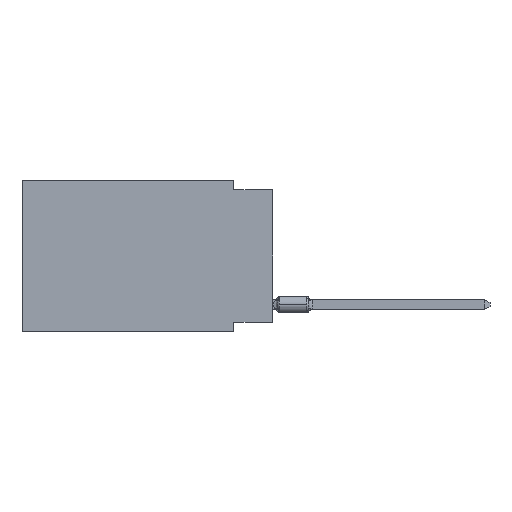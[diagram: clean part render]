
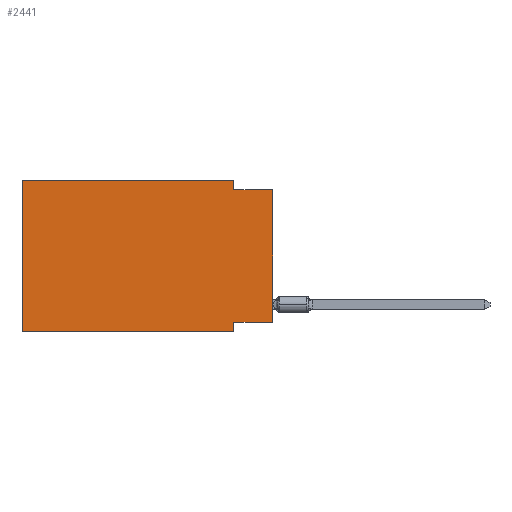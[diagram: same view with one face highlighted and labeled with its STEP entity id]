
A CAD part, left-side view. The second image highlights one B-rep face of the part: STEP entity #2441.
In plain terms, the highlighted planar face has unit normal (-1, 0, 0).
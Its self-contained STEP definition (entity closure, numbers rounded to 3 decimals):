
#49 = CARTESIAN_POINT ( 'NONE',  ( 0., 2.54, 0. ) ) ;
#598 = VECTOR ( 'NONE', #2566, 1000. ) ;
#626 = DIRECTION ( 'NONE',  ( 0., 1., 0. ) ) ;
#1036 = ORIENTED_EDGE ( 'NONE', *, *, #18846, .F. ) ;
#1478 = EDGE_LOOP ( 'NONE', ( #9304, #20825, #6450, #1036, #4518, #3928, #22401, #12254 ) ) ;
#2416 = CARTESIAN_POINT ( 'NONE',  ( 0., 16.383, 0. ) ) ;
#2441 = ADVANCED_FACE ( 'NONE', ( #10969 ), #17260, .F. ) ;
#2447 = CARTESIAN_POINT ( 'NONE',  ( 0., 16.383, -9.906 ) ) ;
#2566 = DIRECTION ( 'NONE',  ( 0., 0., 1. ) ) ;
#2582 = LINE ( 'NONE', #22959, #13742 ) ;
#3321 = DIRECTION ( 'NONE',  ( 0., -1., 0. ) ) ;
#3928 = ORIENTED_EDGE ( 'NONE', *, *, #16907, .T. ) ;
#4476 = VERTEX_POINT ( 'NONE', #7484 ) ;
#4518 = ORIENTED_EDGE ( 'NONE', *, *, #6548, .F. ) ;
#4574 = LINE ( 'NONE', #6696, #598 ) ;
#4639 = VECTOR ( 'NONE', #17729, 1000. ) ;
#4999 = VECTOR ( 'NONE', #14566, 1000. ) ;
#5098 = VERTEX_POINT ( 'NONE', #22165 ) ;
#5389 = LINE ( 'NONE', #21756, #4639 ) ;
#5683 = VECTOR ( 'NONE', #3321, 1000. ) ;
#6090 = EDGE_CURVE ( 'NONE', #9878, #5098, #6742, .T. ) ;
#6450 = ORIENTED_EDGE ( 'NONE', *, *, #26246, .F. ) ;
#6548 = EDGE_CURVE ( 'NONE', #11024, #13679, #7244, .T. ) ;
#6696 = CARTESIAN_POINT ( 'NONE',  ( 0., 0., 0. ) ) ;
#6742 = LINE ( 'NONE', #17210, #25086 ) ;
#6817 = DIRECTION ( 'NONE',  ( 0., -1., 0. ) ) ;
#7244 = LINE ( 'NONE', #23626, #4999 ) ;
#7484 = CARTESIAN_POINT ( 'NONE',  ( 0., 2.54, -0.635 ) ) ;
#7586 = LINE ( 'NONE', #21686, #5683 ) ;
#8890 = VERTEX_POINT ( 'NONE', #19800 ) ;
#9199 = DIRECTION ( 'NONE',  ( 0., 0., -1. ) ) ;
#9304 = ORIENTED_EDGE ( 'NONE', *, *, #19993, .T. ) ;
#9878 = VERTEX_POINT ( 'NONE', #22437 ) ;
#10745 = DIRECTION ( 'NONE',  ( 0., 0., -1. ) ) ;
#10830 = VERTEX_POINT ( 'NONE', #49 ) ;
#10969 = FACE_OUTER_BOUND ( 'NONE', #1478, .T. ) ;
#11024 = VERTEX_POINT ( 'NONE', #2447 ) ;
#12115 = EDGE_CURVE ( 'NONE', #4476, #24833, #5389, .T. ) ;
#12254 = ORIENTED_EDGE ( 'NONE', *, *, #6090, .F. ) ;
#13157 = LINE ( 'NONE', #15167, #19545 ) ;
#13679 = VERTEX_POINT ( 'NONE', #2416 ) ;
#13742 = VECTOR ( 'NONE', #10745, 1000. ) ;
#13767 = LINE ( 'NONE', #15892, #24077 ) ;
#14566 = DIRECTION ( 'NONE',  ( 0., 0., 1. ) ) ;
#15167 = CARTESIAN_POINT ( 'NONE',  ( 0., 16.383, 0. ) ) ;
#15392 = CARTESIAN_POINT ( 'NONE',  ( 0., 16.383, 0. ) ) ;
#15883 = AXIS2_PLACEMENT_3D ( 'NONE', #15392, #25186, #9199 ) ;
#15892 = CARTESIAN_POINT ( 'NONE',  ( 0., 2.54, -9.906 ) ) ;
#16907 = EDGE_CURVE ( 'NONE', #11024, #8890, #7586, .T. ) ;
#17210 = CARTESIAN_POINT ( 'NONE',  ( 0., 0., -9.271 ) ) ;
#17260 = PLANE ( 'NONE',  #15883 ) ;
#17729 = DIRECTION ( 'NONE',  ( 0., -1., 0. ) ) ;
#18846 = EDGE_CURVE ( 'NONE', #13679, #10830, #13157, .T. ) ;
#19545 = VECTOR ( 'NONE', #6817, 1000. ) ;
#19800 = CARTESIAN_POINT ( 'NONE',  ( 0., 2.54, -9.906 ) ) ;
#19904 = DIRECTION ( 'NONE',  ( 0., 0., -1. ) ) ;
#19993 = EDGE_CURVE ( 'NONE', #9878, #24833, #4574, .T. ) ;
#20825 = ORIENTED_EDGE ( 'NONE', *, *, #12115, .F. ) ;
#21686 = CARTESIAN_POINT ( 'NONE',  ( 0., 16.383, -9.906 ) ) ;
#21756 = CARTESIAN_POINT ( 'NONE',  ( 0., 0., -0.635 ) ) ;
#22165 = CARTESIAN_POINT ( 'NONE',  ( 0., 2.54, -9.271 ) ) ;
#22401 = ORIENTED_EDGE ( 'NONE', *, *, #24304, .F. ) ;
#22437 = CARTESIAN_POINT ( 'NONE',  ( 0., 0., -9.271 ) ) ;
#22959 = CARTESIAN_POINT ( 'NONE',  ( 0., 2.54, 0. ) ) ;
#23626 = CARTESIAN_POINT ( 'NONE',  ( 0., 16.383, 0. ) ) ;
#24077 = VECTOR ( 'NONE', #19904, 1000. ) ;
#24304 = EDGE_CURVE ( 'NONE', #5098, #8890, #13767, .T. ) ;
#24679 = CARTESIAN_POINT ( 'NONE',  ( 0., 0., -0.635 ) ) ;
#24833 = VERTEX_POINT ( 'NONE', #24679 ) ;
#25086 = VECTOR ( 'NONE', #626, 1000. ) ;
#25186 = DIRECTION ( 'NONE',  ( 1., 0., 0. ) ) ;
#26246 = EDGE_CURVE ( 'NONE', #10830, #4476, #2582, .T. ) ;
